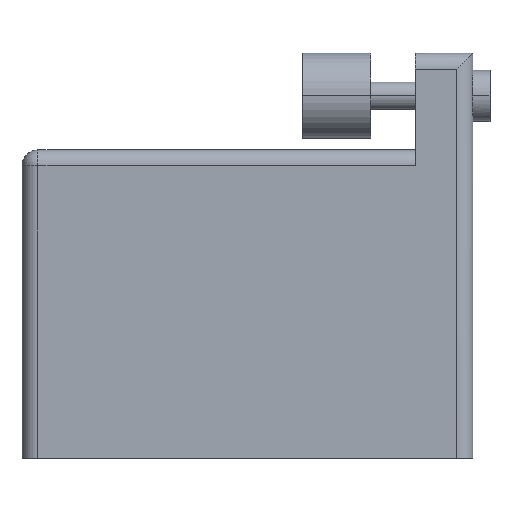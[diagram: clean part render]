
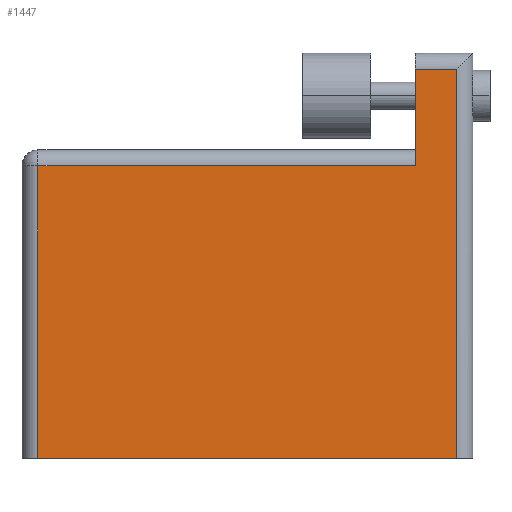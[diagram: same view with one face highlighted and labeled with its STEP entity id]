
A CAD part, top view. The second image highlights one B-rep face of the part: STEP entity #1447.
In plain terms, the highlighted planar face has unit normal (0, 0, 1).
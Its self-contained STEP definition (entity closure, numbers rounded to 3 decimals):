
#15 = VECTOR ( 'NONE', #205, 1000. ) ;
#17 = LINE ( 'NONE', #868, #1563 ) ;
#34 = LINE ( 'NONE', #1769, #15 ) ;
#81 = CARTESIAN_POINT ( 'NONE',  ( 32.461, 30.226, 0. ) ) ;
#182 = CARTESIAN_POINT ( 'NONE',  ( 0., 23.012, 0. ) ) ;
#205 = DIRECTION ( 'NONE',  ( -1., 0., 0. ) ) ;
#330 = AXIS2_PLACEMENT_3D ( 'NONE', #182, #880, #695 ) ;
#333 = VECTOR ( 'NONE', #1161, 1000. ) ;
#519 = DIRECTION ( 'NONE',  ( -1., 0., 0. ) ) ;
#540 = ORIENTED_EDGE ( 'NONE', *, *, #2214, .T. ) ;
#546 = VERTEX_POINT ( 'NONE', #1130 ) ;
#547 = EDGE_LOOP ( 'NONE', ( #1781, #2095, #1403, #1175, #540, #1774 ) ) ;
#596 = CARTESIAN_POINT ( 'NONE',  ( 1.194, 21.819, 0. ) ) ;
#613 = LINE ( 'NONE', #795, #1131 ) ;
#625 = EDGE_CURVE ( 'NONE', #1337, #1174, #613, .T. ) ;
#654 = CARTESIAN_POINT ( 'NONE',  ( 29.337, 30.226, 0. ) ) ;
#668 = CARTESIAN_POINT ( 'NONE',  ( 32.461, 0., 0. ) ) ;
#670 = VERTEX_POINT ( 'NONE', #2201 ) ;
#695 = DIRECTION ( 'NONE',  ( -1., 0., 0. ) ) ;
#795 = CARTESIAN_POINT ( 'NONE',  ( 0., 0., 0. ) ) ;
#868 = CARTESIAN_POINT ( 'NONE',  ( 0., 21.819, 0. ) ) ;
#880 = DIRECTION ( 'NONE',  ( 0., 0., -1. ) ) ;
#925 = VERTEX_POINT ( 'NONE', #596 ) ;
#958 = LINE ( 'NONE', #81, #1899 ) ;
#1022 = CARTESIAN_POINT ( 'NONE',  ( 1.194, 0., 0. ) ) ;
#1025 = CARTESIAN_POINT ( 'NONE',  ( 29.337, 29.032, 0. ) ) ;
#1068 = EDGE_CURVE ( 'NONE', #1174, #546, #958, .T. ) ;
#1123 = DIRECTION ( 'NONE',  ( 0., 1., 0. ) ) ;
#1130 = CARTESIAN_POINT ( 'NONE',  ( 32.461, 29.032, 0. ) ) ;
#1131 = VECTOR ( 'NONE', #1819, 1000. ) ;
#1161 = DIRECTION ( 'NONE',  ( 0., -1., 0. ) ) ;
#1174 = VERTEX_POINT ( 'NONE', #668 ) ;
#1175 = ORIENTED_EDGE ( 'NONE', *, *, #1997, .T. ) ;
#1203 = VERTEX_POINT ( 'NONE', #1025 ) ;
#1327 = VECTOR ( 'NONE', #2002, 1000. ) ;
#1337 = VERTEX_POINT ( 'NONE', #2204 ) ;
#1403 = ORIENTED_EDGE ( 'NONE', *, *, #1535, .T. ) ;
#1447 = ADVANCED_FACE ( 'NONE', ( #1921 ), #1721, .F. ) ;
#1524 = LINE ( 'NONE', #1022, #1327 ) ;
#1535 = EDGE_CURVE ( 'NONE', #546, #1203, #34, .T. ) ;
#1563 = VECTOR ( 'NONE', #519, 1000. ) ;
#1701 = LINE ( 'NONE', #654, #333 ) ;
#1721 = PLANE ( 'NONE',  #330 ) ;
#1769 = CARTESIAN_POINT ( 'NONE',  ( 29.337, 29.032, 0. ) ) ;
#1774 = ORIENTED_EDGE ( 'NONE', *, *, #1984, .T. ) ;
#1781 = ORIENTED_EDGE ( 'NONE', *, *, #625, .T. ) ;
#1819 = DIRECTION ( 'NONE',  ( 1., 0., 0. ) ) ;
#1899 = VECTOR ( 'NONE', #1123, 1000. ) ;
#1921 = FACE_OUTER_BOUND ( 'NONE', #547, .T. ) ;
#1984 = EDGE_CURVE ( 'NONE', #925, #1337, #1524, .T. ) ;
#1997 = EDGE_CURVE ( 'NONE', #1203, #670, #1701, .T. ) ;
#2002 = DIRECTION ( 'NONE',  ( 0., -1., 0. ) ) ;
#2095 = ORIENTED_EDGE ( 'NONE', *, *, #1068, .T. ) ;
#2201 = CARTESIAN_POINT ( 'NONE',  ( 29.337, 21.819, 0. ) ) ;
#2204 = CARTESIAN_POINT ( 'NONE',  ( 1.194, 0., 0. ) ) ;
#2214 = EDGE_CURVE ( 'NONE', #670, #925, #17, .T. ) ;
